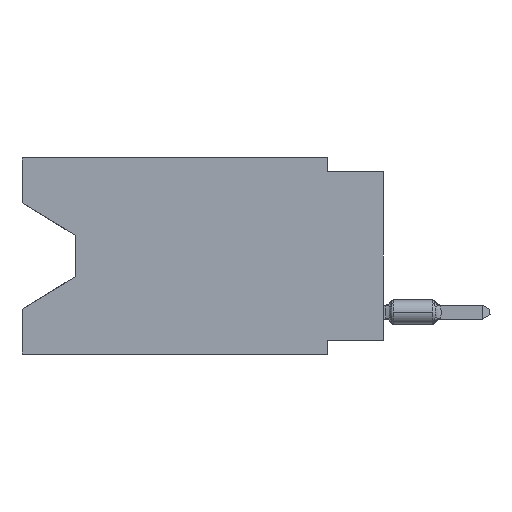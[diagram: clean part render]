
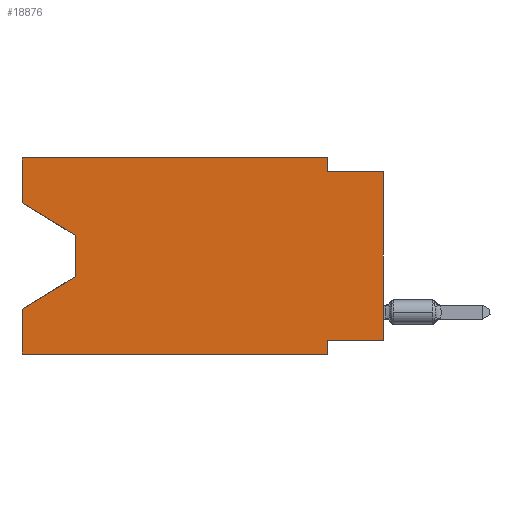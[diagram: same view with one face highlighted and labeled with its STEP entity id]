
A CAD part, left-side view. The second image highlights one B-rep face of the part: STEP entity #18876.
In plain terms, the highlighted planar face has unit normal (-1, 0, 0).
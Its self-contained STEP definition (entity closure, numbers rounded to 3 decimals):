
#308 = VECTOR ( 'NONE', #7564, 1000. ) ;
#754 = ORIENTED_EDGE ( 'NONE', *, *, #18882, .F. ) ;
#1786 = LINE ( 'NONE', #13029, #6212 ) ;
#2723 = CARTESIAN_POINT ( 'NONE',  ( 0., 13.97, -5.385 ) ) ;
#3299 = CARTESIAN_POINT ( 'NONE',  ( 0., 16.383, -2.038 ) ) ;
#3780 = EDGE_CURVE ( 'NONE', #5110, #16541, #1786, .T. ) ;
#3792 = ORIENTED_EDGE ( 'NONE', *, *, #26150, .F. ) ;
#3861 = CARTESIAN_POINT ( 'NONE',  ( 0., 13.97, -3.505 ) ) ;
#4022 = LINE ( 'NONE', #19199, #27005 ) ;
#5110 = VERTEX_POINT ( 'NONE', #6298 ) ;
#5277 = DIRECTION ( 'NONE',  ( 0., 1., 0. ) ) ;
#5339 = EDGE_LOOP ( 'NONE', ( #12346, #11803, #6499, #21269, #14999, #36923, #5956, #20993, #9164, #18298, #754, #3792 ) ) ;
#5956 = ORIENTED_EDGE ( 'NONE', *, *, #34643, .F. ) ;
#6212 = VECTOR ( 'NONE', #33172, 1000. ) ;
#6298 = CARTESIAN_POINT ( 'NONE',  ( 0., 16.383, -8.89 ) ) ;
#6499 = ORIENTED_EDGE ( 'NONE', *, *, #33830, .T. ) ;
#6760 = EDGE_CURVE ( 'NONE', #5110, #21768, #17828, .T. ) ;
#7564 = DIRECTION ( 'NONE',  ( 0., -0.855, -0.519 ) ) ;
#8408 = DIRECTION ( 'NONE',  ( 0., 0., -1. ) ) ;
#8797 = VECTOR ( 'NONE', #8408, 1000. ) ;
#9164 = ORIENTED_EDGE ( 'NONE', *, *, #20042, .F. ) ;
#9531 = LINE ( 'NONE', #10244, #308 ) ;
#9832 = PLANE ( 'NONE',  #20004 ) ;
#9942 = VECTOR ( 'NONE', #17855, 1000. ) ;
#10191 = CARTESIAN_POINT ( 'NONE',  ( 0., 16.383, 0. ) ) ;
#10244 = CARTESIAN_POINT ( 'NONE',  ( 0., 16.383, -2.038 ) ) ;
#10555 = EDGE_CURVE ( 'NONE', #32005, #18286, #16566, .T. ) ;
#10591 = CARTESIAN_POINT ( 'NONE',  ( 0., 2.54, 0. ) ) ;
#10777 = CARTESIAN_POINT ( 'NONE',  ( 0., 2.54, -8.89 ) ) ;
#11573 = CARTESIAN_POINT ( 'NONE',  ( 0., 16.383, -6.852 ) ) ;
#11670 = CARTESIAN_POINT ( 'NONE',  ( 0., 2.54, -8.89 ) ) ;
#11803 = ORIENTED_EDGE ( 'NONE', *, *, #10555, .T. ) ;
#12112 = VECTOR ( 'NONE', #23664, 1000. ) ;
#12288 = EDGE_CURVE ( 'NONE', #18921, #31494, #4022, .T. ) ;
#12346 = ORIENTED_EDGE ( 'NONE', *, *, #14407, .T. ) ;
#12689 = FACE_OUTER_BOUND ( 'NONE', #5339, .T. ) ;
#13029 = CARTESIAN_POINT ( 'NONE',  ( 0., 16.383, 0. ) ) ;
#13472 = CARTESIAN_POINT ( 'NONE',  ( 0., 0., -8.255 ) ) ;
#13507 = LINE ( 'NONE', #33825, #9942 ) ;
#14407 = EDGE_CURVE ( 'NONE', #28615, #32005, #9531, .T. ) ;
#14577 = LINE ( 'NONE', #29019, #32254 ) ;
#14999 = ORIENTED_EDGE ( 'NONE', *, *, #6760, .T. ) ;
#15671 = LINE ( 'NONE', #19244, #26308 ) ;
#16426 = CARTESIAN_POINT ( 'NONE',  ( 0., 0., -8.255 ) ) ;
#16541 = VERTEX_POINT ( 'NONE', #11573 ) ;
#16566 = LINE ( 'NONE', #31593, #8797 ) ;
#16653 = LINE ( 'NONE', #11670, #12112 ) ;
#16719 = VERTEX_POINT ( 'NONE', #10591 ) ;
#17646 = CARTESIAN_POINT ( 'NONE',  ( 0., 13.97, -5.385 ) ) ;
#17828 = LINE ( 'NONE', #35307, #30710 ) ;
#17855 = DIRECTION ( 'NONE',  ( 0., 0., -1. ) ) ;
#18286 = VERTEX_POINT ( 'NONE', #17646 ) ;
#18298 = ORIENTED_EDGE ( 'NONE', *, *, #37494, .F. ) ;
#18734 = DIRECTION ( 'NONE',  ( 0., 0., -1. ) ) ;
#18876 = ADVANCED_FACE ( 'NONE', ( #12689 ), #9832, .F. ) ;
#18882 = EDGE_CURVE ( 'NONE', #29683, #16719, #36200, .T. ) ;
#18921 = VERTEX_POINT ( 'NONE', #16426 ) ;
#19199 = CARTESIAN_POINT ( 'NONE',  ( 0., 0., 0. ) ) ;
#19244 = CARTESIAN_POINT ( 'NONE',  ( 0., 16.383, 0. ) ) ;
#19891 = DIRECTION ( 'NONE',  ( 0., -1., 0. ) ) ;
#20004 = AXIS2_PLACEMENT_3D ( 'NONE', #24625, #30168, #18734 ) ;
#20042 = EDGE_CURVE ( 'NONE', #24038, #31494, #14577, .T. ) ;
#20993 = ORIENTED_EDGE ( 'NONE', *, *, #12288, .T. ) ;
#21269 = ORIENTED_EDGE ( 'NONE', *, *, #3780, .F. ) ;
#21768 = VERTEX_POINT ( 'NONE', #10777 ) ;
#21777 = DIRECTION ( 'NONE',  ( 0., -1., 0. ) ) ;
#23664 = DIRECTION ( 'NONE',  ( 0., 0., -1. ) ) ;
#24038 = VERTEX_POINT ( 'NONE', #31057 ) ;
#24625 = CARTESIAN_POINT ( 'NONE',  ( 0., 16.383, 0. ) ) ;
#26150 = EDGE_CURVE ( 'NONE', #28615, #29683, #15671, .T. ) ;
#26308 = VECTOR ( 'NONE', #33487, 1000. ) ;
#26858 = CARTESIAN_POINT ( 'NONE',  ( 0., 2.54, -8.255 ) ) ;
#27005 = VECTOR ( 'NONE', #33442, 1000. ) ;
#27319 = VECTOR ( 'NONE', #21777, 1000. ) ;
#28615 = VERTEX_POINT ( 'NONE', #3299 ) ;
#28632 = VECTOR ( 'NONE', #31614, 1000. ) ;
#28684 = VECTOR ( 'NONE', #5277, 1000. ) ;
#29019 = CARTESIAN_POINT ( 'NONE',  ( 0., 0., -0.635 ) ) ;
#29436 = DIRECTION ( 'NONE',  ( 0., -1., 0. ) ) ;
#29683 = VERTEX_POINT ( 'NONE', #35110 ) ;
#30168 = DIRECTION ( 'NONE',  ( 1., 0., 0. ) ) ;
#30543 = VERTEX_POINT ( 'NONE', #26858 ) ;
#30710 = VECTOR ( 'NONE', #29436, 1000. ) ;
#31057 = CARTESIAN_POINT ( 'NONE',  ( 0., 2.54, -0.635 ) ) ;
#31494 = VERTEX_POINT ( 'NONE', #33974 ) ;
#31593 = CARTESIAN_POINT ( 'NONE',  ( 0., 13.97, -3.505 ) ) ;
#31614 = DIRECTION ( 'NONE',  ( 0., 0.855, -0.519 ) ) ;
#31862 = EDGE_CURVE ( 'NONE', #30543, #21768, #16653, .T. ) ;
#32005 = VERTEX_POINT ( 'NONE', #3861 ) ;
#32254 = VECTOR ( 'NONE', #19891, 1000. ) ;
#33172 = DIRECTION ( 'NONE',  ( 0., 0., 1. ) ) ;
#33442 = DIRECTION ( 'NONE',  ( 0., 0., 1. ) ) ;
#33487 = DIRECTION ( 'NONE',  ( 0., 0., 1. ) ) ;
#33598 = LINE ( 'NONE', #13472, #28684 ) ;
#33825 = CARTESIAN_POINT ( 'NONE',  ( 0., 2.54, 0. ) ) ;
#33830 = EDGE_CURVE ( 'NONE', #18286, #16541, #34451, .T. ) ;
#33974 = CARTESIAN_POINT ( 'NONE',  ( 0., 0., -0.635 ) ) ;
#34451 = LINE ( 'NONE', #2723, #28632 ) ;
#34643 = EDGE_CURVE ( 'NONE', #18921, #30543, #33598, .T. ) ;
#35110 = CARTESIAN_POINT ( 'NONE',  ( 0., 16.383, 0. ) ) ;
#35307 = CARTESIAN_POINT ( 'NONE',  ( 0., 16.383, -8.89 ) ) ;
#36200 = LINE ( 'NONE', #10191, #27319 ) ;
#36923 = ORIENTED_EDGE ( 'NONE', *, *, #31862, .F. ) ;
#37494 = EDGE_CURVE ( 'NONE', #16719, #24038, #13507, .T. ) ;
